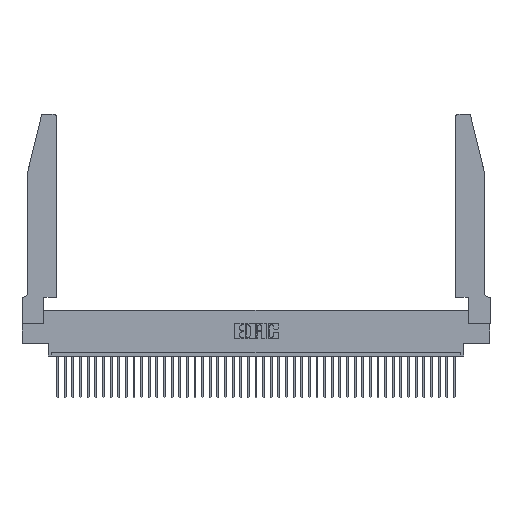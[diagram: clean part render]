
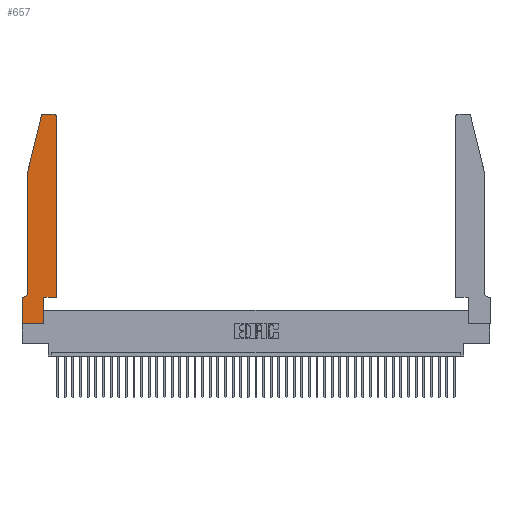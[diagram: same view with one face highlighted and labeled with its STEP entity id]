
A CAD part, top view. The second image highlights one B-rep face of the part: STEP entity #657.
In plain terms, the highlighted planar face has unit normal (0, 0, 1).
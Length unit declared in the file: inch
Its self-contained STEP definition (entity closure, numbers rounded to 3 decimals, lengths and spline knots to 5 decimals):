
#657 = ADVANCED_FACE ( 'NONE', ( #20581 ), #17592, .T. ) ;
#863 = CARTESIAN_POINT ( 'NONE',  ( 0., 0.35, 0.37 ) ) ;
#870 = VERTEX_POINT ( 'NONE', #20746 ) ;
#944 = EDGE_CURVE ( 'NONE', #29060, #2650, #16377, .T. ) ;
#1150 = DIRECTION ( 'NONE',  ( 1., 0., 0. ) ) ;
#1546 = CARTESIAN_POINT ( 'NONE',  ( 0.2605, 2.75, 0.37 ) ) ;
#1757 = VERTEX_POINT ( 'NONE', #37133 ) ;
#2140 = AXIS2_PLACEMENT_3D ( 'NONE', #37380, #17441, #1150 ) ;
#2432 = VECTOR ( 'NONE', #8054, 39.37008 ) ;
#2650 = VERTEX_POINT ( 'NONE', #35593 ) ;
#2731 = EDGE_LOOP ( 'NONE', ( #6649, #30323, #24267, #31062, #41069, #11226, #33167, #6831, #37210, #6293, #12561, #28576 ) ) ;
#3812 = AXIS2_PLACEMENT_3D ( 'NONE', #22094, #39057, #41816 ) ;
#3850 = DIRECTION ( 'NONE',  ( 0., 1., 0. ) ) ;
#4397 = EDGE_CURVE ( 'NONE', #26857, #6169, #28084, .T. ) ;
#4530 = CARTESIAN_POINT ( 'NONE',  ( 0., 0., 0.37 ) ) ;
#5467 = CARTESIAN_POINT ( 'NONE',  ( 0.0055, 0.42, 0.37 ) ) ;
#6049 = CARTESIAN_POINT ( 'NONE',  ( 0.0755, 0.35, 0.37 ) ) ;
#6169 = VERTEX_POINT ( 'NONE', #28124 ) ;
#6293 = ORIENTED_EDGE ( 'NONE', *, *, #4397, .T. ) ;
#6382 = CARTESIAN_POINT ( 'NONE',  ( 0.2865, 0.35, 0.37 ) ) ;
#6649 = ORIENTED_EDGE ( 'NONE', *, *, #24445, .T. ) ;
#6831 = ORIENTED_EDGE ( 'NONE', *, *, #31078, .T. ) ;
#7440 = VECTOR ( 'NONE', #27938, 39.37008 ) ;
#7826 = LINE ( 'NONE', #20522, #20393 ) ;
#7950 = CARTESIAN_POINT ( 'NONE',  ( 0.0755, 2., 0.37 ) ) ;
#8054 = DIRECTION ( 'NONE',  ( 1., 0., 0. ) ) ;
#8158 = EDGE_CURVE ( 'NONE', #32067, #870, #17365, .T. ) ;
#8471 = DIRECTION ( 'NONE',  ( -0.239, -0.971, 0. ) ) ;
#8689 = CIRCLE ( 'NONE', #3812, 0.03 ) ;
#10010 = DIRECTION ( 'NONE',  ( 1., 0., 0. ) ) ;
#11226 = ORIENTED_EDGE ( 'NONE', *, *, #11313, .T. ) ;
#11313 = EDGE_CURVE ( 'NONE', #29707, #29060, #20225, .T. ) ;
#11958 = CARTESIAN_POINT ( 'NONE',  ( 0.25487, 2.72718, 0.37 ) ) ;
#12561 = ORIENTED_EDGE ( 'NONE', *, *, #40364, .T. ) ;
#12748 = AXIS2_PLACEMENT_3D ( 'NONE', #16320, #33367, #10010 ) ;
#13511 = VECTOR ( 'NONE', #35603, 39.37008 ) ;
#13652 = CARTESIAN_POINT ( 'NONE',  ( 0.2865, 0.35, 0.37 ) ) ;
#13987 = LINE ( 'NONE', #7950, #35938 ) ;
#14310 = CARTESIAN_POINT ( 'NONE',  ( 0.4205, 2.75, 0.37 ) ) ;
#14428 = DIRECTION ( 'NONE',  ( -1., 0., 0. ) ) ;
#16047 = CARTESIAN_POINT ( 'NONE',  ( 0.0055, 0.35, 0.37 ) ) ;
#16320 = CARTESIAN_POINT ( 'NONE',  ( 0.4205, 2.72, 0.37 ) ) ;
#16377 = LINE ( 'NONE', #4530, #7440 ) ;
#17056 = DIRECTION ( 'NONE',  ( 0., 1., 0. ) ) ;
#17365 = LINE ( 'NONE', #17880, #40841 ) ;
#17441 = DIRECTION ( 'NONE',  ( 0., 0., 1. ) ) ;
#17592 = PLANE ( 'NONE',  #2140 ) ;
#17791 = VECTOR ( 'NONE', #14428, 39.37008 ) ;
#17865 = AXIS2_PLACEMENT_3D ( 'NONE', #5467, #35543, #31730 ) ;
#17880 = CARTESIAN_POINT ( 'NONE',  ( 0.0755, 2., 0.37 ) ) ;
#18852 = CARTESIAN_POINT ( 'NONE',  ( 0., 0., 0.37 ) ) ;
#20225 = LINE ( 'NONE', #6049, #36894 ) ;
#20393 = VECTOR ( 'NONE', #3850, 39.37008 ) ;
#20522 = CARTESIAN_POINT ( 'NONE',  ( 0.4505, 0.35, 0.37 ) ) ;
#20581 = FACE_OUTER_BOUND ( 'NONE', #2731, .T. ) ;
#20746 = CARTESIAN_POINT ( 'NONE',  ( 0.0755, 2., 0.37 ) ) ;
#21096 = CARTESIAN_POINT ( 'NONE',  ( 0.0755, 0.42, 0.37 ) ) ;
#21632 = VERTEX_POINT ( 'NONE', #39771 ) ;
#22094 = CARTESIAN_POINT ( 'NONE',  ( 0.284, 2.72, 0.37 ) ) ;
#22771 = EDGE_CURVE ( 'NONE', #25573, #26857, #30962, .T. ) ;
#24267 = ORIENTED_EDGE ( 'NONE', *, *, #8158, .T. ) ;
#24445 = EDGE_CURVE ( 'NONE', #24649, #1757, #37582, .T. ) ;
#24526 = VERTEX_POINT ( 'NONE', #21096 ) ;
#24649 = VERTEX_POINT ( 'NONE', #14310 ) ;
#25573 = VERTEX_POINT ( 'NONE', #38857 ) ;
#26179 = CIRCLE ( 'NONE', #17865, 0.07 ) ;
#26857 = VERTEX_POINT ( 'NONE', #13652 ) ;
#27938 = DIRECTION ( 'NONE',  ( 0., -1., 0. ) ) ;
#28084 = LINE ( 'NONE', #28111, #2432 ) ;
#28111 = CARTESIAN_POINT ( 'NONE',  ( 0.4505, 0.35, 0.37 ) ) ;
#28124 = CARTESIAN_POINT ( 'NONE',  ( 0.4505, 0.35, 0.37 ) ) ;
#28576 = ORIENTED_EDGE ( 'NONE', *, *, #40227, .T. ) ;
#29060 = VERTEX_POINT ( 'NONE', #863 ) ;
#29421 = DIRECTION ( 'NONE',  ( -1., 0., 0. ) ) ;
#29707 = VERTEX_POINT ( 'NONE', #16047 ) ;
#29956 = VECTOR ( 'NONE', #17056, 39.37008 ) ;
#30323 = ORIENTED_EDGE ( 'NONE', *, *, #42349, .T. ) ;
#30962 = LINE ( 'NONE', #6382, #29956 ) ;
#31062 = ORIENTED_EDGE ( 'NONE', *, *, #34252, .T. ) ;
#31078 = EDGE_CURVE ( 'NONE', #2650, #25573, #42245, .T. ) ;
#31730 = DIRECTION ( 'NONE',  ( -1., 0., 0. ) ) ;
#32067 = VERTEX_POINT ( 'NONE', #11958 ) ;
#32790 = EDGE_CURVE ( 'NONE', #24526, #29707, #26179, .T. ) ;
#33167 = ORIENTED_EDGE ( 'NONE', *, *, #944, .T. ) ;
#33367 = DIRECTION ( 'NONE',  ( 0., 0., 1. ) ) ;
#34252 = EDGE_CURVE ( 'NONE', #870, #24526, #13987, .T. ) ;
#34815 = DIRECTION ( 'NONE',  ( 0., -1., 0. ) ) ;
#35543 = DIRECTION ( 'NONE',  ( 0., 0., -1. ) ) ;
#35593 = CARTESIAN_POINT ( 'NONE',  ( 0., 0., 0.37 ) ) ;
#35603 = DIRECTION ( 'NONE',  ( 1., 0., 0. ) ) ;
#35938 = VECTOR ( 'NONE', #34815, 39.37008 ) ;
#36894 = VECTOR ( 'NONE', #29421, 39.37008 ) ;
#37133 = CARTESIAN_POINT ( 'NONE',  ( 0.284, 2.75, 0.37 ) ) ;
#37210 = ORIENTED_EDGE ( 'NONE', *, *, #22771, .T. ) ;
#37380 = CARTESIAN_POINT ( 'NONE',  ( 0., 0.35, 0.37 ) ) ;
#37582 = LINE ( 'NONE', #1546, #17791 ) ;
#38857 = CARTESIAN_POINT ( 'NONE',  ( 0.2865, 0., 0.37 ) ) ;
#39057 = DIRECTION ( 'NONE',  ( 0., 0., 1. ) ) ;
#39771 = CARTESIAN_POINT ( 'NONE',  ( 0.4505, 2.72, 0.37 ) ) ;
#40227 = EDGE_CURVE ( 'NONE', #21632, #24649, #40730, .T. ) ;
#40364 = EDGE_CURVE ( 'NONE', #6169, #21632, #7826, .T. ) ;
#40730 = CIRCLE ( 'NONE', #12748, 0.03 ) ;
#40841 = VECTOR ( 'NONE', #8471, 39.37008 ) ;
#41069 = ORIENTED_EDGE ( 'NONE', *, *, #32790, .T. ) ;
#41816 = DIRECTION ( 'NONE',  ( 1., 0., 0. ) ) ;
#42245 = LINE ( 'NONE', #18852, #13511 ) ;
#42349 = EDGE_CURVE ( 'NONE', #1757, #32067, #8689, .T. ) ;
